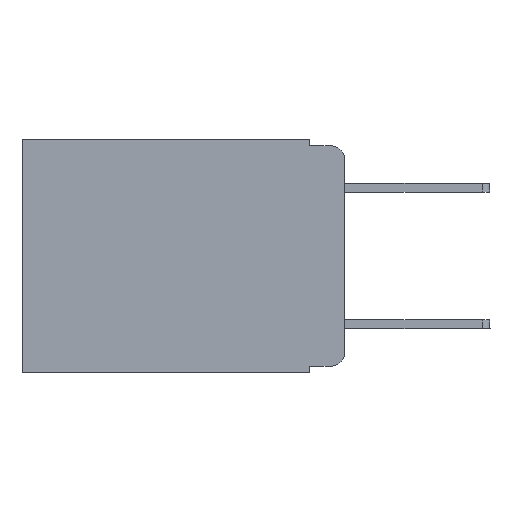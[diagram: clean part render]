
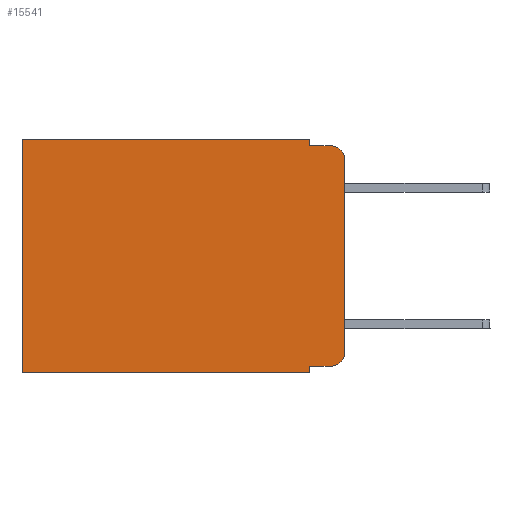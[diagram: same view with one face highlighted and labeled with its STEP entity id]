
A CAD part, left-side view. The second image highlights one B-rep face of the part: STEP entity #15541.
In plain terms, the highlighted planar face has unit normal (-1, 0, 0).
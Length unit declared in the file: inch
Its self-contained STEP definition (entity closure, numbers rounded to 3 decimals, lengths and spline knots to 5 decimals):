
#134 = VERTEX_POINT ( 'NONE', #8056 ) ;
#205 = EDGE_CURVE ( 'NONE', #1528, #22203, #13991, .T. ) ;
#673 = CARTESIAN_POINT ( 'NONE',  ( 0.298, 0., 0. ) ) ;
#1311 = LINE ( 'NONE', #21474, #11808 ) ;
#1528 = VERTEX_POINT ( 'NONE', #15547 ) ;
#1556 = CARTESIAN_POINT ( 'NONE',  ( 0.298, 0., 0. ) ) ;
#1953 = VERTEX_POINT ( 'NONE', #22840 ) ;
#2489 = PLANE ( 'NONE',  #18815 ) ;
#2794 = EDGE_CURVE ( 'NONE', #21337, #1953, #7338, .T. ) ;
#3611 = VERTEX_POINT ( 'NONE', #7245 ) ;
#3814 = ORIENTED_EDGE ( 'NONE', *, *, #11024, .T. ) ;
#3879 = DIRECTION ( 'NONE',  ( 0., 0., -1. ) ) ;
#4361 = LINE ( 'NONE', #14478, #17614 ) ;
#4374 = ORIENTED_EDGE ( 'NONE', *, *, #23279, .F. ) ;
#4487 = VECTOR ( 'NONE', #9738, 39.37008 ) ;
#4595 = ORIENTED_EDGE ( 'NONE', *, *, #2794, .T. ) ;
#4992 = DIRECTION ( 'NONE',  ( 0., 0., -1. ) ) ;
#5184 = EDGE_CURVE ( 'NONE', #21915, #1528, #21581, .T. ) ;
#5593 = CARTESIAN_POINT ( 'NONE',  ( 0.298, 0., -0.343 ) ) ;
#6202 = CARTESIAN_POINT ( 'NONE',  ( 0.298, 0.473, 0. ) ) ;
#6434 = VERTEX_POINT ( 'NONE', #10908 ) ;
#6813 = VECTOR ( 'NONE', #24552, 39.37008 ) ;
#7047 = ORIENTED_EDGE ( 'NONE', *, *, #18928, .F. ) ;
#7089 = CARTESIAN_POINT ( 'NONE',  ( 0.298, 0.051, 0. ) ) ;
#7136 = ORIENTED_EDGE ( 'NONE', *, *, #20819, .F. ) ;
#7245 = CARTESIAN_POINT ( 'NONE',  ( 0.298, 0.051, -0.01 ) ) ;
#7338 = LINE ( 'NONE', #21623, #11567 ) ;
#8056 = CARTESIAN_POINT ( 'NONE',  ( 0.298, 0.02, -0.01 ) ) ;
#8528 = DIRECTION ( 'NONE',  ( -1., 0., 0. ) ) ;
#9045 = LINE ( 'NONE', #7089, #12229 ) ;
#9065 = ORIENTED_EDGE ( 'NONE', *, *, #205, .T. ) ;
#9539 = DIRECTION ( 'NONE',  ( 0., -1., 0. ) ) ;
#9738 = DIRECTION ( 'NONE',  ( 0., 1., 0. ) ) ;
#10564 = DIRECTION ( 'NONE',  ( 1., 0., 0. ) ) ;
#10614 = DIRECTION ( 'NONE',  ( 0., -1., 0. ) ) ;
#10908 = CARTESIAN_POINT ( 'NONE',  ( 0.298, 0., -0.313 ) ) ;
#11024 = EDGE_CURVE ( 'NONE', #12965, #134, #12951, .T. ) ;
#11567 = VECTOR ( 'NONE', #9539, 39.37008 ) ;
#11808 = VECTOR ( 'NONE', #3879, 39.37008 ) ;
#12229 = VECTOR ( 'NONE', #4992, 39.37008 ) ;
#12247 = FACE_OUTER_BOUND ( 'NONE', #12736, .T. ) ;
#12736 = EDGE_LOOP ( 'NONE', ( #15012, #3814, #7136, #22878, #16091, #9065, #4374, #7047, #4595, #22483 ) ) ;
#12745 = DIRECTION ( 'NONE',  ( -1., 0., 0. ) ) ;
#12951 = CIRCLE ( 'NONE', #16228, 0.02 ) ;
#12965 = VERTEX_POINT ( 'NONE', #25108 ) ;
#13502 = DIRECTION ( 'NONE',  ( 0., 1., 0. ) ) ;
#13679 = LINE ( 'NONE', #23342, #6813 ) ;
#13887 = EDGE_CURVE ( 'NONE', #21915, #3611, #9045, .T. ) ;
#13991 = LINE ( 'NONE', #6202, #24172 ) ;
#14478 = CARTESIAN_POINT ( 'NONE',  ( 0.298, 0.051, -0.01 ) ) ;
#15012 = ORIENTED_EDGE ( 'NONE', *, *, #17916, .F. ) ;
#15067 = CARTESIAN_POINT ( 'NONE',  ( 0.298, 0.02, -0.03 ) ) ;
#15081 = EDGE_CURVE ( 'NONE', #1953, #6434, #25439, .T. ) ;
#15541 = ADVANCED_FACE ( 'NONE', ( #12247 ), #2489, .F. ) ;
#15547 = CARTESIAN_POINT ( 'NONE',  ( 0.298, 0.473, 0. ) ) ;
#16091 = ORIENTED_EDGE ( 'NONE', *, *, #5184, .T. ) ;
#16228 = AXIS2_PLACEMENT_3D ( 'NONE', #15067, #12745, #20578 ) ;
#16232 = CARTESIAN_POINT ( 'NONE',  ( 0.298, 0.051, -0.333 ) ) ;
#16507 = CARTESIAN_POINT ( 'NONE',  ( 0.298, 0.02, -0.313 ) ) ;
#17614 = VECTOR ( 'NONE', #10614, 39.37008 ) ;
#17916 = EDGE_CURVE ( 'NONE', #12965, #6434, #13679, .T. ) ;
#18379 = DIRECTION ( 'NONE',  ( 0., 0., -1. ) ) ;
#18815 = AXIS2_PLACEMENT_3D ( 'NONE', #673, #10564, #18379 ) ;
#18928 = EDGE_CURVE ( 'NONE', #21337, #19185, #1311, .T. ) ;
#19185 = VERTEX_POINT ( 'NONE', #22352 ) ;
#20070 = AXIS2_PLACEMENT_3D ( 'NONE', #16507, #8528, #20233 ) ;
#20233 = DIRECTION ( 'NONE',  ( 0., 0., -1. ) ) ;
#20578 = DIRECTION ( 'NONE',  ( 0., 0., -1. ) ) ;
#20819 = EDGE_CURVE ( 'NONE', #3611, #134, #4361, .T. ) ;
#21224 = LINE ( 'NONE', #5593, #22209 ) ;
#21337 = VERTEX_POINT ( 'NONE', #16232 ) ;
#21474 = CARTESIAN_POINT ( 'NONE',  ( 0.298, 0.051, 0. ) ) ;
#21575 = CARTESIAN_POINT ( 'NONE',  ( 0.298, 0.051, 0. ) ) ;
#21581 = LINE ( 'NONE', #1556, #4487 ) ;
#21623 = CARTESIAN_POINT ( 'NONE',  ( 0.298, 0.051, -0.333 ) ) ;
#21833 = DIRECTION ( 'NONE',  ( 0., 0., -1. ) ) ;
#21915 = VERTEX_POINT ( 'NONE', #21575 ) ;
#22203 = VERTEX_POINT ( 'NONE', #22849 ) ;
#22209 = VECTOR ( 'NONE', #13502, 39.37008 ) ;
#22352 = CARTESIAN_POINT ( 'NONE',  ( 0.298, 0.051, -0.343 ) ) ;
#22483 = ORIENTED_EDGE ( 'NONE', *, *, #15081, .T. ) ;
#22840 = CARTESIAN_POINT ( 'NONE',  ( 0.298, 0.02, -0.333 ) ) ;
#22849 = CARTESIAN_POINT ( 'NONE',  ( 0.298, 0.473, -0.343 ) ) ;
#22878 = ORIENTED_EDGE ( 'NONE', *, *, #13887, .F. ) ;
#23279 = EDGE_CURVE ( 'NONE', #19185, #22203, #21224, .T. ) ;
#23342 = CARTESIAN_POINT ( 'NONE',  ( 0.298, 0., 0. ) ) ;
#24172 = VECTOR ( 'NONE', #21833, 39.37008 ) ;
#24552 = DIRECTION ( 'NONE',  ( 0., 0., -1. ) ) ;
#25108 = CARTESIAN_POINT ( 'NONE',  ( 0.298, 0., -0.03 ) ) ;
#25439 = CIRCLE ( 'NONE', #20070, 0.02 ) ;
